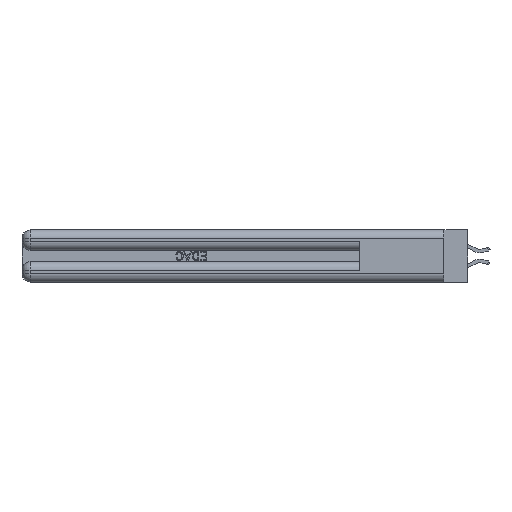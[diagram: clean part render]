
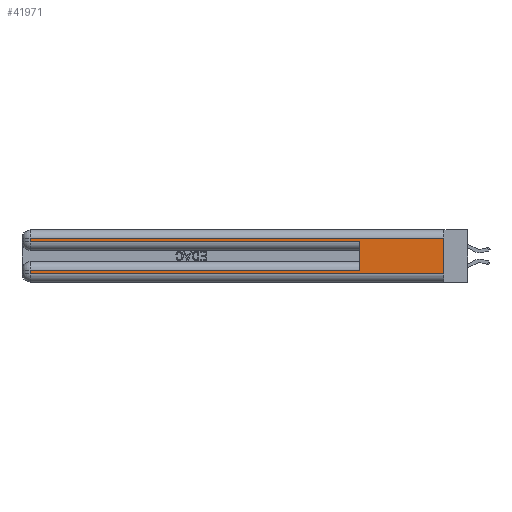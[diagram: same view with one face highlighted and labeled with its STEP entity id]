
A CAD part, left-side view. The second image highlights one B-rep face of the part: STEP entity #41971.
In plain terms, the highlighted planar face has unit normal (-1, 0, 0).
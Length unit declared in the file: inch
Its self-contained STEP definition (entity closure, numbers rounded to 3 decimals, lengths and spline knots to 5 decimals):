
#953 = DIRECTION ( 'NONE',  ( 0., 0., -1. ) ) ;
#1773 = CARTESIAN_POINT ( 'NONE',  ( 0., 0.6, 0.145 ) ) ;
#2127 = LINE ( 'NONE', #37918, #19971 ) ;
#2210 = DIRECTION ( 'NONE',  ( 0., -1., 0. ) ) ;
#2279 = LINE ( 'NONE', #1773, #11320 ) ;
#2488 = DIRECTION ( 'NONE',  ( 0., 0., -1. ) ) ;
#3843 = ORIENTED_EDGE ( 'NONE', *, *, #24481, .F. ) ;
#4705 = VERTEX_POINT ( 'NONE', #29215 ) ;
#4832 = VERTEX_POINT ( 'NONE', #26007 ) ;
#4994 = CARTESIAN_POINT ( 'NONE',  ( 0., 0.6, 0.085 ) ) ;
#5110 = ORIENTED_EDGE ( 'NONE', *, *, #39248, .T. ) ;
#5524 = ORIENTED_EDGE ( 'NONE', *, *, #41316, .T. ) ;
#8092 = DIRECTION ( 'NONE',  ( 0., 0., -1. ) ) ;
#8731 = EDGE_CURVE ( 'NONE', #4832, #15574, #22021, .T. ) ;
#9945 = EDGE_CURVE ( 'NONE', #30858, #48096, #42028, .T. ) ;
#11320 = VECTOR ( 'NONE', #16997, 39.37008 ) ;
#13275 = VECTOR ( 'NONE', #8092, 39.37008 ) ;
#15122 = DIRECTION ( 'NONE',  ( 0., -1., 0. ) ) ;
#15549 = EDGE_CURVE ( 'NONE', #37946, #15574, #29591, .T. ) ;
#15574 = VERTEX_POINT ( 'NONE', #40882 ) ;
#15582 = ORIENTED_EDGE ( 'NONE', *, *, #24274, .T. ) ;
#16061 = VECTOR ( 'NONE', #2210, 39.37008 ) ;
#16915 = EDGE_LOOP ( 'NONE', ( #19754, #5110, #15582, #5524, #3843, #45424, #27133, #36336 ) ) ;
#16997 = DIRECTION ( 'NONE',  ( 0., 0., 1. ) ) ;
#19612 = DIRECTION ( 'NONE',  ( 0., 0., -1. ) ) ;
#19754 = ORIENTED_EDGE ( 'NONE', *, *, #8731, .F. ) ;
#19971 = VECTOR ( 'NONE', #19612, 39.37008 ) ;
#20436 = CARTESIAN_POINT ( 'NONE',  ( 0., 2.94, 0.06 ) ) ;
#20969 = VECTOR ( 'NONE', #15122, 39.37008 ) ;
#21044 = CARTESIAN_POINT ( 'NONE',  ( 0., 0., 0.37 ) ) ;
#21559 = LINE ( 'NONE', #23619, #39937 ) ;
#22021 = LINE ( 'NONE', #30377, #13275 ) ;
#22433 = CARTESIAN_POINT ( 'NONE',  ( 0., 2.94, 0.31 ) ) ;
#23619 = CARTESIAN_POINT ( 'NONE',  ( 0., 2.94, 0.37 ) ) ;
#24274 = EDGE_CURVE ( 'NONE', #26748, #41957, #2127, .T. ) ;
#24481 = EDGE_CURVE ( 'NONE', #30858, #4705, #2279, .T. ) ;
#24813 = VECTOR ( 'NONE', #46509, 39.37008 ) ;
#25068 = DIRECTION ( 'NONE',  ( 1., 0., 0. ) ) ;
#26007 = CARTESIAN_POINT ( 'NONE',  ( 0., 0., 0.31 ) ) ;
#26748 = VERTEX_POINT ( 'NONE', #22433 ) ;
#27133 = ORIENTED_EDGE ( 'NONE', *, *, #28105, .T. ) ;
#28105 = EDGE_CURVE ( 'NONE', #48096, #37946, #21559, .T. ) ;
#28606 = PLANE ( 'NONE',  #39781 ) ;
#29215 = CARTESIAN_POINT ( 'NONE',  ( 0., 0.6, 0.285 ) ) ;
#29591 = LINE ( 'NONE', #37188, #20969 ) ;
#30377 = CARTESIAN_POINT ( 'NONE',  ( 0., 0., 0.37 ) ) ;
#30858 = VERTEX_POINT ( 'NONE', #4994 ) ;
#32231 = VECTOR ( 'NONE', #40929, 39.37008 ) ;
#32301 = CARTESIAN_POINT ( 'NONE',  ( 0., 2.94, 0.285 ) ) ;
#35588 = LINE ( 'NONE', #46809, #16061 ) ;
#35735 = LINE ( 'NONE', #42811, #24813 ) ;
#36336 = ORIENTED_EDGE ( 'NONE', *, *, #15549, .T. ) ;
#37188 = CARTESIAN_POINT ( 'NONE',  ( 0., 0., 0.06 ) ) ;
#37918 = CARTESIAN_POINT ( 'NONE',  ( 0., 2.94, 0.37 ) ) ;
#37946 = VERTEX_POINT ( 'NONE', #20436 ) ;
#39248 = EDGE_CURVE ( 'NONE', #4832, #26748, #35735, .T. ) ;
#39781 = AXIS2_PLACEMENT_3D ( 'NONE', #21044, #25068, #2488 ) ;
#39937 = VECTOR ( 'NONE', #953, 39.37008 ) ;
#40882 = CARTESIAN_POINT ( 'NONE',  ( 0., 0., 0.06 ) ) ;
#40929 = DIRECTION ( 'NONE',  ( 0., 1., 0. ) ) ;
#41316 = EDGE_CURVE ( 'NONE', #41957, #4705, #35588, .T. ) ;
#41957 = VERTEX_POINT ( 'NONE', #32301 ) ;
#41971 = ADVANCED_FACE ( 'NONE', ( #45891 ), #28606, .F. ) ;
#42028 = LINE ( 'NONE', #48138, #32231 ) ;
#42811 = CARTESIAN_POINT ( 'NONE',  ( 0., 0., 0.31 ) ) ;
#44510 = CARTESIAN_POINT ( 'NONE',  ( 0., 2.94, 0.085 ) ) ;
#45424 = ORIENTED_EDGE ( 'NONE', *, *, #9945, .T. ) ;
#45891 = FACE_OUTER_BOUND ( 'NONE', #16915, .T. ) ;
#46509 = DIRECTION ( 'NONE',  ( 0., 1., 0. ) ) ;
#46809 = CARTESIAN_POINT ( 'NONE',  ( 0., 0., 0.285 ) ) ;
#48096 = VERTEX_POINT ( 'NONE', #44510 ) ;
#48138 = CARTESIAN_POINT ( 'NONE',  ( 0., 0., 0.085 ) ) ;
